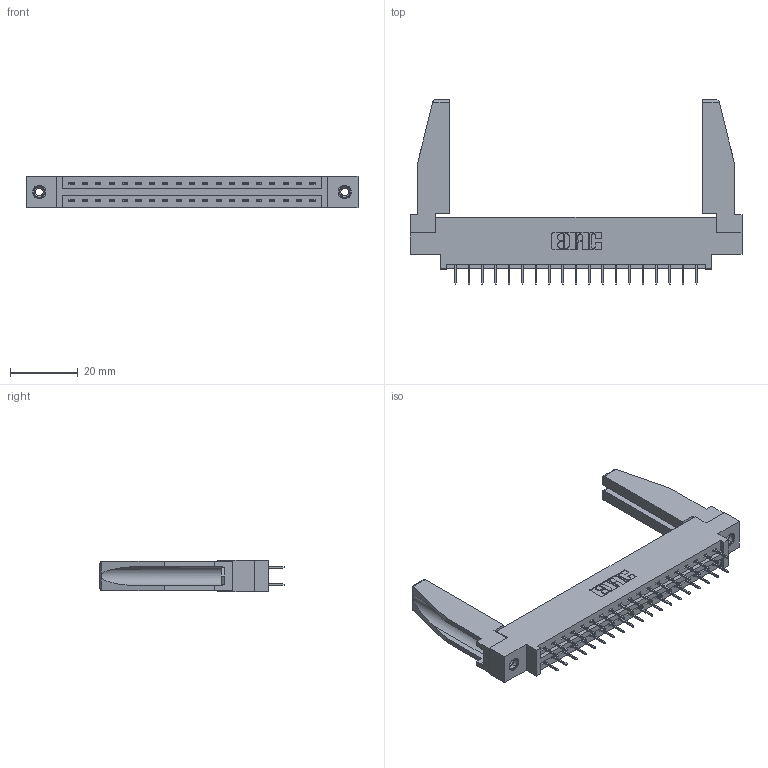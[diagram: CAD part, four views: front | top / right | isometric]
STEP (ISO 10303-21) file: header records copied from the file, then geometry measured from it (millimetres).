
FILE_DESCRIPTION (( 'STEP AP203' ), '1' );
FILE_NAME ('337-038-524-878.STEP', '2019-10-11T11:19:46', ( '' ), ( '' ), 'SwSTEP 2.0', 'SolidWorks 2016', '' );
FILE_SCHEMA (( 'CONFIG_CONTROL_DESIGN' ));
Length unit declared in the file: inch
Products named in the file (5): 307-220-078; 337-038-524-878; 337 Part_0.170 Offset - 0.156 Dia-TI; 345-292-001_345-293-124; 345-250-001_345-250-001-102
Assembly tree (43 placements, depth 2):
  337-038-524-878
    337 Part_0.170 Offset - 0.156 Dia-TI
    345-292-001_345-293-124  x38
    345-250-001_345-250-001-102  x2
    307-220-078  x2
Bounding box: 98.3 x 54.49 x 9.4 mm (x, y, z)
Volume: 13871.6 mm3; surface area: 14704.2 mm2
Topology: 43 solids, 43 shells, 2452 faces, 6923 edges, 4454 vertices
Faces by surface type: plane 1830, cylinder 606, cone 12, torus 4
Entity records: 20352 total; most frequent: CARTESIAN_POINT 3448, ORIENTED_EDGE 3340, DIRECTION 2982, EDGE_CURVE 1670, LINE 1508, VECTOR 1508, VERTEX_POINT 1104, AXIS2_PLACEMENT_3D 737
